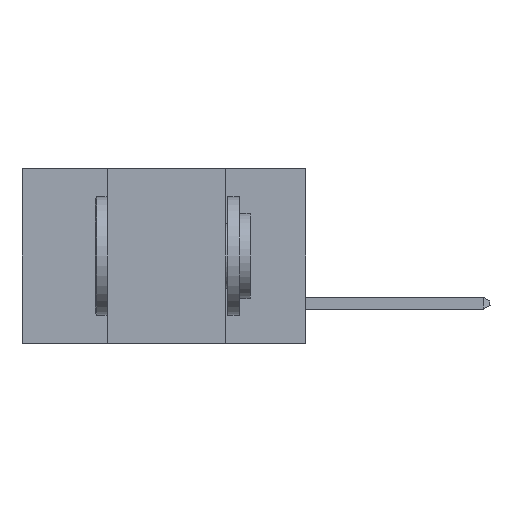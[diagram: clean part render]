
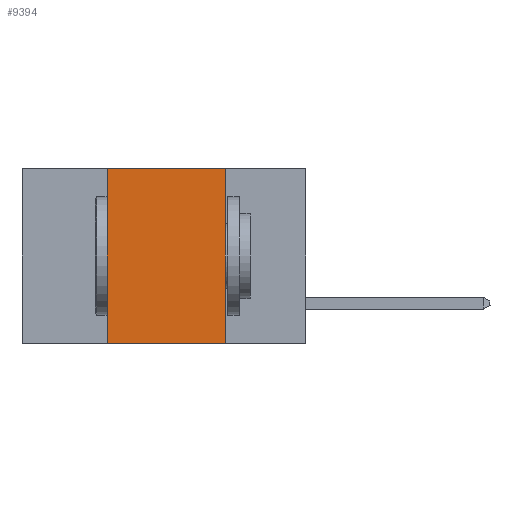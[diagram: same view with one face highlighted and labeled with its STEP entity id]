
A CAD part, left-side view. The second image highlights one B-rep face of the part: STEP entity #9394.
In plain terms, the highlighted planar face has unit normal (-1, 0, 0).
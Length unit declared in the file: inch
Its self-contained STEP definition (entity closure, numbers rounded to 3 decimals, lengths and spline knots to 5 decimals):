
#231 = CARTESIAN_POINT ( 'NONE',  ( 0., 0.42, 0. ) ) ;
#406 = ORIENTED_EDGE ( 'NONE', *, *, #6097, .F. ) ;
#535 = LINE ( 'NONE', #13686, #3313 ) ;
#721 = DIRECTION ( 'NONE',  ( 0., -1., 0. ) ) ;
#1463 = VECTOR ( 'NONE', #1552, 39.37008 ) ;
#1552 = DIRECTION ( 'NONE',  ( 0., 0., 1. ) ) ;
#2568 = LINE ( 'NONE', #6631, #9447 ) ;
#3269 = CARTESIAN_POINT ( 'NONE',  ( 0., 0.6, 0. ) ) ;
#3313 = VECTOR ( 'NONE', #721, 39.37008 ) ;
#3369 = DIRECTION ( 'NONE',  ( 0., -1., 0. ) ) ;
#3507 = VERTEX_POINT ( 'NONE', #4783 ) ;
#4206 = LINE ( 'NONE', #3269, #11652 ) ;
#4374 = EDGE_CURVE ( 'NONE', #13697, #10340, #535, .T. ) ;
#4783 = CARTESIAN_POINT ( 'NONE',  ( 0., 0.17, 0. ) ) ;
#5068 = ORIENTED_EDGE ( 'NONE', *, *, #15316, .F. ) ;
#5163 = VERTEX_POINT ( 'NONE', #9398 ) ;
#5485 = AXIS2_PLACEMENT_3D ( 'NONE', #6752, #7958, #11581 ) ;
#5662 = EDGE_LOOP ( 'NONE', ( #12329, #406, #5068, #14496 ) ) ;
#5682 = LINE ( 'NONE', #231, #1463 ) ;
#6097 = EDGE_CURVE ( 'NONE', #5163, #3507, #4206, .T. ) ;
#6543 = EDGE_CURVE ( 'NONE', #3507, #10340, #2568, .T. ) ;
#6631 = CARTESIAN_POINT ( 'NONE',  ( 0., 0.17, 0. ) ) ;
#6752 = CARTESIAN_POINT ( 'NONE',  ( 0., 0.6, 0. ) ) ;
#7958 = DIRECTION ( 'NONE',  ( 1., 0., 0. ) ) ;
#8957 = DIRECTION ( 'NONE',  ( 0., 0., -1. ) ) ;
#9394 = ADVANCED_FACE ( 'NONE', ( #14893 ), #12872, .F. ) ;
#9398 = CARTESIAN_POINT ( 'NONE',  ( 0., 0.42, 0. ) ) ;
#9447 = VECTOR ( 'NONE', #8957, 39.37008 ) ;
#10340 = VERTEX_POINT ( 'NONE', #10530 ) ;
#10530 = CARTESIAN_POINT ( 'NONE',  ( 0., 0.17, -0.37 ) ) ;
#11581 = DIRECTION ( 'NONE',  ( 0., 0., -1. ) ) ;
#11652 = VECTOR ( 'NONE', #3369, 39.37008 ) ;
#12329 = ORIENTED_EDGE ( 'NONE', *, *, #6543, .F. ) ;
#12872 = PLANE ( 'NONE',  #5485 ) ;
#13686 = CARTESIAN_POINT ( 'NONE',  ( 0., 0.6, -0.37 ) ) ;
#13697 = VERTEX_POINT ( 'NONE', #15191 ) ;
#14496 = ORIENTED_EDGE ( 'NONE', *, *, #4374, .T. ) ;
#14893 = FACE_OUTER_BOUND ( 'NONE', #5662, .T. ) ;
#15191 = CARTESIAN_POINT ( 'NONE',  ( 0., 0.42, -0.37 ) ) ;
#15316 = EDGE_CURVE ( 'NONE', #13697, #5163, #5682, .T. ) ;
